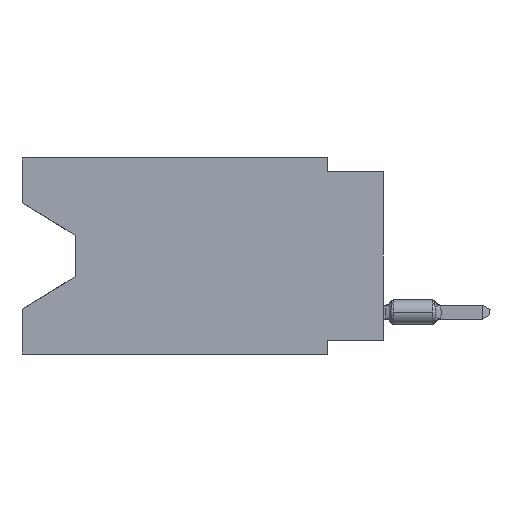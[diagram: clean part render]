
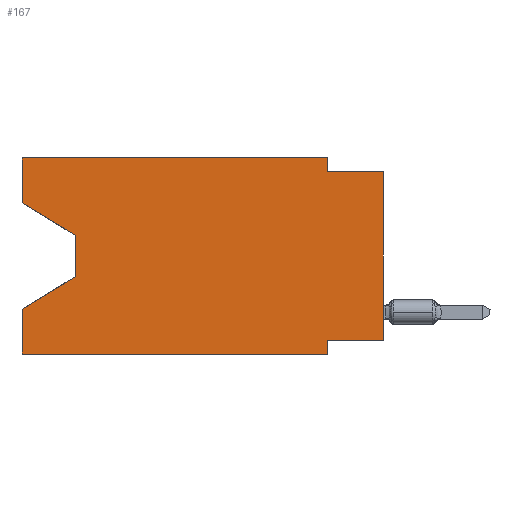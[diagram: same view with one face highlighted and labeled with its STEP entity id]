
A CAD part, left-side view. The second image highlights one B-rep face of the part: STEP entity #167.
In plain terms, the highlighted planar face has unit normal (-1, 0, 0).
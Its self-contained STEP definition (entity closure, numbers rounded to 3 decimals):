
#45 = CARTESIAN_POINT ( 'NONE',  ( 0., 2.54, -8.89 ) ) ;
#167 = ADVANCED_FACE ( 'NONE', ( #17726 ), #23380, .F. ) ;
#211 = EDGE_CURVE ( 'NONE', #7219, #3971, #21903, .T. ) ;
#231 = CARTESIAN_POINT ( 'NONE',  ( 0., 16.383, 0. ) ) ;
#392 = LINE ( 'NONE', #17259, #12649 ) ;
#621 = DIRECTION ( 'NONE',  ( 0., 0.855, -0.519 ) ) ;
#633 = CARTESIAN_POINT ( 'NONE',  ( 0., 16.383, -8.89 ) ) ;
#2187 = DIRECTION ( 'NONE',  ( 0., 0., -1. ) ) ;
#2193 = VERTEX_POINT ( 'NONE', #8360 ) ;
#2312 = ORIENTED_EDGE ( 'NONE', *, *, #24119, .F. ) ;
#2472 = DIRECTION ( 'NONE',  ( 0., 0., -1. ) ) ;
#2813 = CARTESIAN_POINT ( 'NONE',  ( 0., 2.54, 0. ) ) ;
#2866 = EDGE_CURVE ( 'NONE', #14780, #6390, #20911, .T. ) ;
#3086 = DIRECTION ( 'NONE',  ( 0., -1., 0. ) ) ;
#3591 = LINE ( 'NONE', #14924, #23448 ) ;
#3839 = DIRECTION ( 'NONE',  ( 0., 0., 1. ) ) ;
#3971 = VERTEX_POINT ( 'NONE', #20586 ) ;
#4004 = VERTEX_POINT ( 'NONE', #45 ) ;
#4447 = CARTESIAN_POINT ( 'NONE',  ( 0., 16.383, 0. ) ) ;
#4694 = LINE ( 'NONE', #21434, #12315 ) ;
#5717 = EDGE_CURVE ( 'NONE', #19389, #17086, #10946, .T. ) ;
#6174 = CARTESIAN_POINT ( 'NONE',  ( 0., 16.383, -2.038 ) ) ;
#6390 = VERTEX_POINT ( 'NONE', #18122 ) ;
#6391 = LINE ( 'NONE', #14030, #15033 ) ;
#7219 = VERTEX_POINT ( 'NONE', #23119 ) ;
#7380 = EDGE_CURVE ( 'NONE', #17086, #7219, #19049, .T. ) ;
#7476 = ORIENTED_EDGE ( 'NONE', *, *, #16494, .T. ) ;
#7744 = CARTESIAN_POINT ( 'NONE',  ( 0., 16.383, -2.038 ) ) ;
#7807 = ORIENTED_EDGE ( 'NONE', *, *, #7868, .T. ) ;
#7816 = VERTEX_POINT ( 'NONE', #6174 ) ;
#7868 = EDGE_CURVE ( 'NONE', #16559, #14780, #4694, .T. ) ;
#7949 = CARTESIAN_POINT ( 'NONE',  ( 0., 2.54, -8.255 ) ) ;
#8255 = DIRECTION ( 'NONE',  ( 0., 0., 1. ) ) ;
#8360 = CARTESIAN_POINT ( 'NONE',  ( 0., 16.383, -8.89 ) ) ;
#8840 = CARTESIAN_POINT ( 'NONE',  ( 0., 2.54, -8.89 ) ) ;
#9330 = VERTEX_POINT ( 'NONE', #7949 ) ;
#10064 = VECTOR ( 'NONE', #3086, 1000. ) ;
#10576 = EDGE_LOOP ( 'NONE', ( #14731, #7807, #17977, #21679, #7476, #2312, #23949, #13825, #10801, #16903, #18348, #16790 ) ) ;
#10801 = ORIENTED_EDGE ( 'NONE', *, *, #211, .F. ) ;
#10946 = LINE ( 'NONE', #231, #18548 ) ;
#11145 = VECTOR ( 'NONE', #21884, 1000. ) ;
#11358 = EDGE_CURVE ( 'NONE', #22042, #9330, #6391, .T. ) ;
#11816 = CARTESIAN_POINT ( 'NONE',  ( 0., 16.383, 0. ) ) ;
#12315 = VECTOR ( 'NONE', #19700, 1000. ) ;
#12424 = VECTOR ( 'NONE', #2187, 1000. ) ;
#12649 = VECTOR ( 'NONE', #15653, 1000. ) ;
#12984 = CARTESIAN_POINT ( 'NONE',  ( 0., 13.97, -5.385 ) ) ;
#13825 = ORIENTED_EDGE ( 'NONE', *, *, #20889, .T. ) ;
#14030 = CARTESIAN_POINT ( 'NONE',  ( 0., 0., -8.255 ) ) ;
#14105 = CARTESIAN_POINT ( 'NONE',  ( 0., 0., -8.255 ) ) ;
#14731 = ORIENTED_EDGE ( 'NONE', *, *, #22624, .T. ) ;
#14780 = VERTEX_POINT ( 'NONE', #12984 ) ;
#14924 = CARTESIAN_POINT ( 'NONE',  ( 0., 0., 0. ) ) ;
#15033 = VECTOR ( 'NONE', #21520, 1000. ) ;
#15286 = DIRECTION ( 'NONE',  ( 0., -1., 0. ) ) ;
#15653 = DIRECTION ( 'NONE',  ( 0., 0., 1. ) ) ;
#16494 = EDGE_CURVE ( 'NONE', #2193, #4004, #19459, .T. ) ;
#16496 = EDGE_CURVE ( 'NONE', #2193, #6390, #392, .T. ) ;
#16559 = VERTEX_POINT ( 'NONE', #21049 ) ;
#16720 = VECTOR ( 'NONE', #621, 1000. ) ;
#16790 = ORIENTED_EDGE ( 'NONE', *, *, #19406, .F. ) ;
#16903 = ORIENTED_EDGE ( 'NONE', *, *, #7380, .F. ) ;
#17086 = VERTEX_POINT ( 'NONE', #2813 ) ;
#17118 = LINE ( 'NONE', #7744, #22192 ) ;
#17232 = DIRECTION ( 'NONE',  ( 0., -0.855, -0.519 ) ) ;
#17239 = VECTOR ( 'NONE', #8255, 1000. ) ;
#17259 = CARTESIAN_POINT ( 'NONE',  ( 0., 16.383, 0. ) ) ;
#17726 = FACE_OUTER_BOUND ( 'NONE', #10576, .T. ) ;
#17977 = ORIENTED_EDGE ( 'NONE', *, *, #2866, .T. ) ;
#18122 = CARTESIAN_POINT ( 'NONE',  ( 0., 16.383, -6.852 ) ) ;
#18348 = ORIENTED_EDGE ( 'NONE', *, *, #5717, .F. ) ;
#18458 = DIRECTION ( 'NONE',  ( 0., -1., 0. ) ) ;
#18548 = VECTOR ( 'NONE', #18458, 1000. ) ;
#19049 = LINE ( 'NONE', #20752, #12424 ) ;
#19329 = DIRECTION ( 'NONE',  ( 1., 0., 0. ) ) ;
#19389 = VERTEX_POINT ( 'NONE', #22544 ) ;
#19406 = EDGE_CURVE ( 'NONE', #7816, #19389, #21302, .T. ) ;
#19459 = LINE ( 'NONE', #633, #20879 ) ;
#19700 = DIRECTION ( 'NONE',  ( 0., 0., -1. ) ) ;
#20036 = LINE ( 'NONE', #8840, #11145 ) ;
#20586 = CARTESIAN_POINT ( 'NONE',  ( 0., 0., -0.635 ) ) ;
#20752 = CARTESIAN_POINT ( 'NONE',  ( 0., 2.54, 0. ) ) ;
#20879 = VECTOR ( 'NONE', #15286, 1000. ) ;
#20889 = EDGE_CURVE ( 'NONE', #22042, #3971, #3591, .T. ) ;
#20911 = LINE ( 'NONE', #21159, #16720 ) ;
#21049 = CARTESIAN_POINT ( 'NONE',  ( 0., 13.97, -3.505 ) ) ;
#21159 = CARTESIAN_POINT ( 'NONE',  ( 0., 13.97, -5.385 ) ) ;
#21302 = LINE ( 'NONE', #4447, #17239 ) ;
#21434 = CARTESIAN_POINT ( 'NONE',  ( 0., 13.97, -3.505 ) ) ;
#21520 = DIRECTION ( 'NONE',  ( 0., 1., 0. ) ) ;
#21679 = ORIENTED_EDGE ( 'NONE', *, *, #16496, .F. ) ;
#21884 = DIRECTION ( 'NONE',  ( 0., 0., -1. ) ) ;
#21903 = LINE ( 'NONE', #24104, #10064 ) ;
#22042 = VERTEX_POINT ( 'NONE', #14105 ) ;
#22192 = VECTOR ( 'NONE', #17232, 1000. ) ;
#22544 = CARTESIAN_POINT ( 'NONE',  ( 0., 16.383, 0. ) ) ;
#22624 = EDGE_CURVE ( 'NONE', #7816, #16559, #17118, .T. ) ;
#22999 = AXIS2_PLACEMENT_3D ( 'NONE', #11816, #19329, #2472 ) ;
#23119 = CARTESIAN_POINT ( 'NONE',  ( 0., 2.54, -0.635 ) ) ;
#23380 = PLANE ( 'NONE',  #22999 ) ;
#23448 = VECTOR ( 'NONE', #3839, 1000. ) ;
#23949 = ORIENTED_EDGE ( 'NONE', *, *, #11358, .F. ) ;
#24104 = CARTESIAN_POINT ( 'NONE',  ( 0., 0., -0.635 ) ) ;
#24119 = EDGE_CURVE ( 'NONE', #9330, #4004, #20036, .T. ) ;
